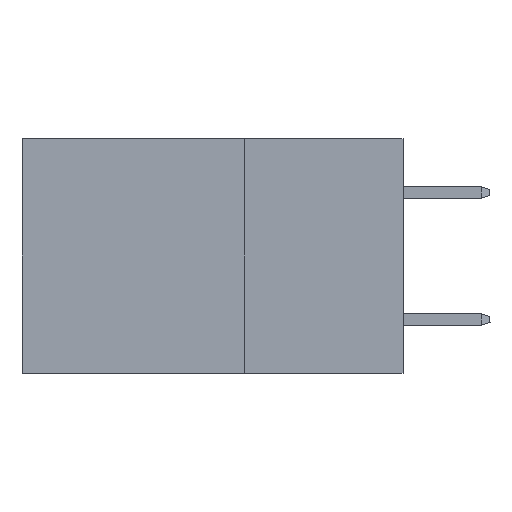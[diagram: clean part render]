
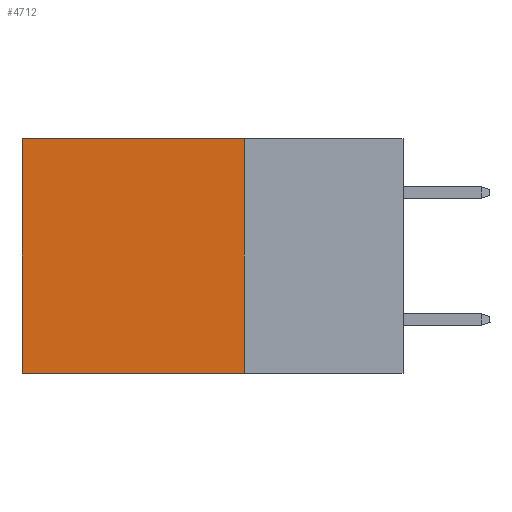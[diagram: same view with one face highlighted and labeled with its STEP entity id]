
A CAD part, left-side view. The second image highlights one B-rep face of the part: STEP entity #4712.
In plain terms, the highlighted planar face has unit normal (-1, 0, 0).
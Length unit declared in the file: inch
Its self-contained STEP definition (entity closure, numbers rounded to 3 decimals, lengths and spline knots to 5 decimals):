
#579 = CARTESIAN_POINT ( 'NONE',  ( 0.2875, 0.6, 0. ) ) ;
#654 = CARTESIAN_POINT ( 'NONE',  ( 0.2875, 0.6, -0.37 ) ) ;
#715 = CARTESIAN_POINT ( 'NONE',  ( 0.2875, 0.25, 0. ) ) ;
#829 = CARTESIAN_POINT ( 'NONE',  ( 0.2875, 0.25, 0. ) ) ;
#1533 = VERTEX_POINT ( 'NONE', #715 ) ;
#2278 = CARTESIAN_POINT ( 'NONE',  ( 0.2875, 0.25, 0. ) ) ;
#4608 = VERTEX_POINT ( 'NONE', #579 ) ;
#4712 = ADVANCED_FACE ( 'NONE', ( #14684 ), #24388, .F. ) ;
#5812 = CARTESIAN_POINT ( 'NONE',  ( 0.2875, 0.25, 0. ) ) ;
#6163 = EDGE_LOOP ( 'NONE', ( #24764, #10078, #7601, #17559 ) ) ;
#7601 = ORIENTED_EDGE ( 'NONE', *, *, #19011, .F. ) ;
#7761 = EDGE_CURVE ( 'NONE', #10899, #16520, #14656, .T. ) ;
#9742 = LINE ( 'NONE', #5812, #16405 ) ;
#10027 = DIRECTION ( 'NONE',  ( 0., 1., 0. ) ) ;
#10078 = ORIENTED_EDGE ( 'NONE', *, *, #7761, .F. ) ;
#10899 = VERTEX_POINT ( 'NONE', #19182 ) ;
#11261 = DIRECTION ( 'NONE',  ( 0., 0., -1. ) ) ;
#11327 = AXIS2_PLACEMENT_3D ( 'NONE', #829, #18667, #14199 ) ;
#12220 = EDGE_CURVE ( 'NONE', #1533, #4608, #19725, .T. ) ;
#13582 = CARTESIAN_POINT ( 'NONE',  ( 0.2875, 0.6, 0. ) ) ;
#14132 = EDGE_CURVE ( 'NONE', #4608, #16520, #15483, .T. ) ;
#14199 = DIRECTION ( 'NONE',  ( 0., 0., -1. ) ) ;
#14656 = LINE ( 'NONE', #22447, #18333 ) ;
#14684 = FACE_OUTER_BOUND ( 'NONE', #6163, .T. ) ;
#15483 = LINE ( 'NONE', #13582, #18490 ) ;
#15613 = DIRECTION ( 'NONE',  ( 0., 0., -1. ) ) ;
#16405 = VECTOR ( 'NONE', #11261, 39.37008 ) ;
#16520 = VERTEX_POINT ( 'NONE', #654 ) ;
#16837 = VECTOR ( 'NONE', #10027, 39.37008 ) ;
#17559 = ORIENTED_EDGE ( 'NONE', *, *, #12220, .T. ) ;
#18333 = VECTOR ( 'NONE', #20658, 39.37008 ) ;
#18490 = VECTOR ( 'NONE', #15613, 39.37008 ) ;
#18667 = DIRECTION ( 'NONE',  ( 1., 0., 0. ) ) ;
#19011 = EDGE_CURVE ( 'NONE', #1533, #10899, #9742, .T. ) ;
#19182 = CARTESIAN_POINT ( 'NONE',  ( 0.2875, 0.25, -0.37 ) ) ;
#19725 = LINE ( 'NONE', #2278, #16837 ) ;
#20658 = DIRECTION ( 'NONE',  ( 0., 1., 0. ) ) ;
#22447 = CARTESIAN_POINT ( 'NONE',  ( 0.2875, 0.25, -0.37 ) ) ;
#24388 = PLANE ( 'NONE',  #11327 ) ;
#24764 = ORIENTED_EDGE ( 'NONE', *, *, #14132, .T. ) ;
